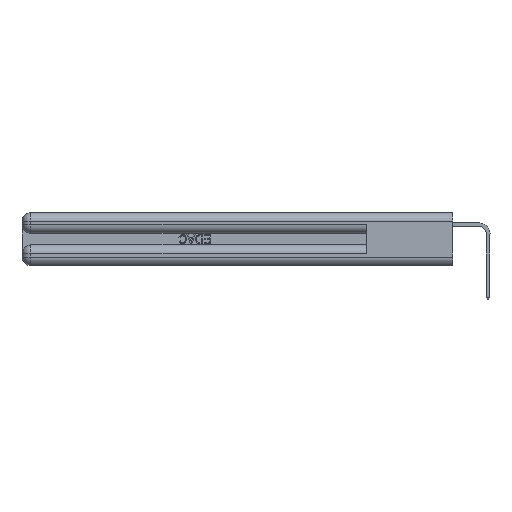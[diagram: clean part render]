
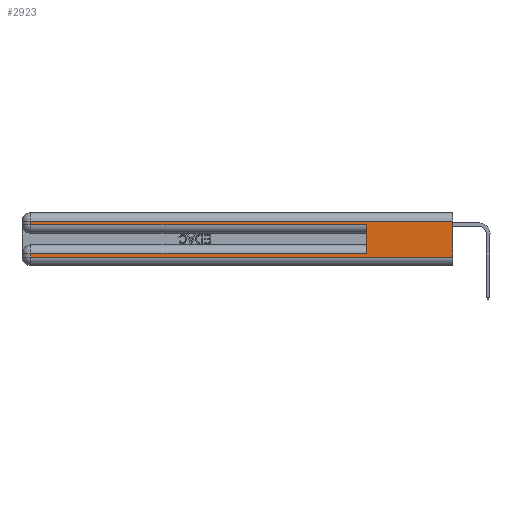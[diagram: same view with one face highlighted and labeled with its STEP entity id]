
A CAD part, left-side view. The second image highlights one B-rep face of the part: STEP entity #2923.
In plain terms, the highlighted planar face has unit normal (-1, 0, 0).
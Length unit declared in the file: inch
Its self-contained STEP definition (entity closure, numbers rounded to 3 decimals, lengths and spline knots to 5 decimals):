
#70 = DIRECTION ( 'NONE',  ( 0., 0., -1. ) ) ;
#1261 = LINE ( 'NONE', #9068, #31641 ) ;
#2097 = LINE ( 'NONE', #6450, #24460 ) ;
#2923 = ADVANCED_FACE ( 'NONE', ( #20217 ), #22172, .F. ) ;
#3037 = EDGE_CURVE ( 'NONE', #19343, #5210, #7370, .T. ) ;
#3101 = ORIENTED_EDGE ( 'NONE', *, *, #19218, .T. ) ;
#4104 = VERTEX_POINT ( 'NONE', #13448 ) ;
#4242 = LINE ( 'NONE', #14131, #21356 ) ;
#4857 = CARTESIAN_POINT ( 'NONE',  ( 0., 2.94, 0.37 ) ) ;
#4911 = ORIENTED_EDGE ( 'NONE', *, *, #30123, .F. ) ;
#4937 = CARTESIAN_POINT ( 'NONE',  ( 0., 2.94, 0.06 ) ) ;
#5210 = VERTEX_POINT ( 'NONE', #22024 ) ;
#5284 = LINE ( 'NONE', #37576, #36615 ) ;
#6149 = VERTEX_POINT ( 'NONE', #4937 ) ;
#6450 = CARTESIAN_POINT ( 'NONE',  ( 0., 0., 0.06 ) ) ;
#7018 = DIRECTION ( 'NONE',  ( 1., 0., 0. ) ) ;
#7370 = LINE ( 'NONE', #26451, #38672 ) ;
#8050 = EDGE_LOOP ( 'NONE', ( #19044, #15856, #23222, #18838, #4911, #3101, #30845, #35619 ) ) ;
#8718 = AXIS2_PLACEMENT_3D ( 'NONE', #37116, #7018, #28306 ) ;
#9068 = CARTESIAN_POINT ( 'NONE',  ( 0., 0.6, 0.145 ) ) ;
#10388 = VECTOR ( 'NONE', #13118, 39.37008 ) ;
#10481 = VECTOR ( 'NONE', #70, 39.37008 ) ;
#10611 = VECTOR ( 'NONE', #26166, 39.37008 ) ;
#11296 = DIRECTION ( 'NONE',  ( 0., -1., 0. ) ) ;
#12222 = CARTESIAN_POINT ( 'NONE',  ( 0., 2.94, 0.37 ) ) ;
#13118 = DIRECTION ( 'NONE',  ( 0., 1., 0. ) ) ;
#13448 = CARTESIAN_POINT ( 'NONE',  ( 0., 0.6, 0.085 ) ) ;
#14131 = CARTESIAN_POINT ( 'NONE',  ( 0., 0., 0.085 ) ) ;
#14830 = VERTEX_POINT ( 'NONE', #33959 ) ;
#15014 = DIRECTION ( 'NONE',  ( 0., 0., 1. ) ) ;
#15527 = EDGE_CURVE ( 'NONE', #22616, #14830, #5284, .T. ) ;
#15856 = ORIENTED_EDGE ( 'NONE', *, *, #33869, .T. ) ;
#16379 = DIRECTION ( 'NONE',  ( 0., 0., -1. ) ) ;
#16473 = EDGE_CURVE ( 'NONE', #19882, #6149, #18526, .T. ) ;
#17039 = DIRECTION ( 'NONE',  ( 0., 1., 0. ) ) ;
#17083 = VERTEX_POINT ( 'NONE', #21855 ) ;
#18526 = LINE ( 'NONE', #12222, #10481 ) ;
#18662 = LINE ( 'NONE', #4857, #10611 ) ;
#18838 = ORIENTED_EDGE ( 'NONE', *, *, #3037, .T. ) ;
#19044 = ORIENTED_EDGE ( 'NONE', *, *, #15527, .F. ) ;
#19071 = CARTESIAN_POINT ( 'NONE',  ( 0., 0., 0.31 ) ) ;
#19218 = EDGE_CURVE ( 'NONE', #4104, #19882, #4242, .T. ) ;
#19343 = VERTEX_POINT ( 'NONE', #26930 ) ;
#19882 = VERTEX_POINT ( 'NONE', #20978 ) ;
#20217 = FACE_OUTER_BOUND ( 'NONE', #8050, .T. ) ;
#20978 = CARTESIAN_POINT ( 'NONE',  ( 0., 2.94, 0.085 ) ) ;
#21356 = VECTOR ( 'NONE', #17039, 39.37008 ) ;
#21596 = DIRECTION ( 'NONE',  ( 0., -1., 0. ) ) ;
#21855 = CARTESIAN_POINT ( 'NONE',  ( 0., 2.94, 0.31 ) ) ;
#22024 = CARTESIAN_POINT ( 'NONE',  ( 0., 0.6, 0.285 ) ) ;
#22172 = PLANE ( 'NONE',  #8718 ) ;
#22616 = VERTEX_POINT ( 'NONE', #39229 ) ;
#23042 = EDGE_CURVE ( 'NONE', #17083, #19343, #18662, .T. ) ;
#23222 = ORIENTED_EDGE ( 'NONE', *, *, #23042, .T. ) ;
#24460 = VECTOR ( 'NONE', #21596, 39.37008 ) ;
#25190 = EDGE_CURVE ( 'NONE', #6149, #14830, #2097, .T. ) ;
#26166 = DIRECTION ( 'NONE',  ( 0., 0., -1. ) ) ;
#26451 = CARTESIAN_POINT ( 'NONE',  ( 0., 0., 0.285 ) ) ;
#26559 = LINE ( 'NONE', #19071, #10388 ) ;
#26930 = CARTESIAN_POINT ( 'NONE',  ( 0., 2.94, 0.285 ) ) ;
#28306 = DIRECTION ( 'NONE',  ( 0., 0., -1. ) ) ;
#30123 = EDGE_CURVE ( 'NONE', #4104, #5210, #1261, .T. ) ;
#30845 = ORIENTED_EDGE ( 'NONE', *, *, #16473, .T. ) ;
#31641 = VECTOR ( 'NONE', #15014, 39.37008 ) ;
#33869 = EDGE_CURVE ( 'NONE', #22616, #17083, #26559, .T. ) ;
#33959 = CARTESIAN_POINT ( 'NONE',  ( 0., 0., 0.06 ) ) ;
#35619 = ORIENTED_EDGE ( 'NONE', *, *, #25190, .T. ) ;
#36615 = VECTOR ( 'NONE', #16379, 39.37008 ) ;
#37116 = CARTESIAN_POINT ( 'NONE',  ( 0., 0., 0.37 ) ) ;
#37576 = CARTESIAN_POINT ( 'NONE',  ( 0., 0., 0.37 ) ) ;
#38672 = VECTOR ( 'NONE', #11296, 39.37008 ) ;
#39229 = CARTESIAN_POINT ( 'NONE',  ( 0., 0., 0.31 ) ) ;
